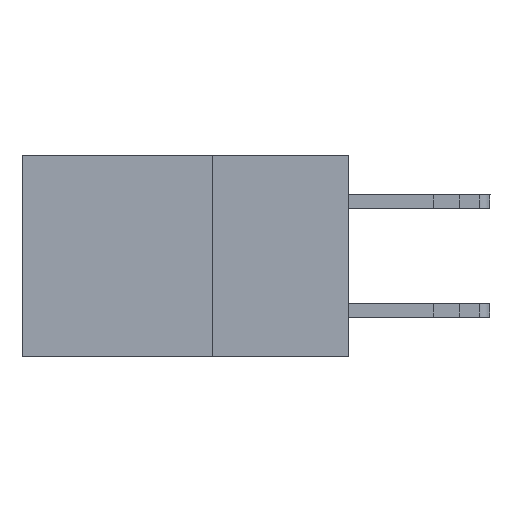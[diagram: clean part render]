
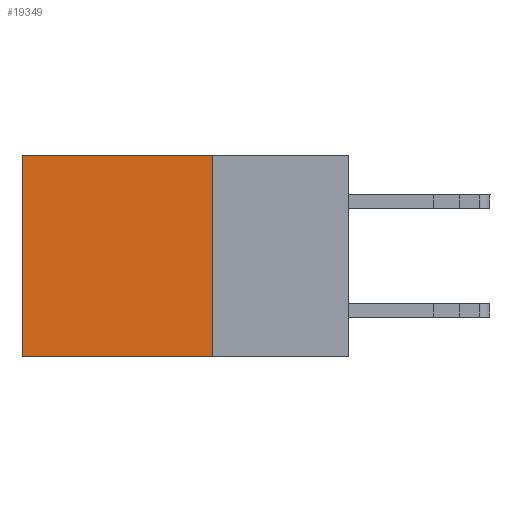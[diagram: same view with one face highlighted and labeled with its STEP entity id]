
A CAD part, left-side view. The second image highlights one B-rep face of the part: STEP entity #19349.
In plain terms, the highlighted planar face has unit normal (-1, 0, 0).
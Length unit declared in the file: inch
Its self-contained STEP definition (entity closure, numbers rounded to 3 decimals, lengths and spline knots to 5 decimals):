
#587 = DIRECTION ( 'NONE',  ( 0., 0., -1. ) ) ;
#704 = EDGE_CURVE ( 'NONE', #1761, #6371, #3309, .T. ) ;
#825 = LINE ( 'NONE', #7078, #16611 ) ;
#1733 = ORIENTED_EDGE ( 'NONE', *, *, #9300, .F. ) ;
#1761 = VERTEX_POINT ( 'NONE', #5199 ) ;
#2770 = LINE ( 'NONE', #9032, #12662 ) ;
#3309 = LINE ( 'NONE', #9355, #19589 ) ;
#5199 = CARTESIAN_POINT ( 'NONE',  ( 0.298, 0.6, 0. ) ) ;
#5217 = PLANE ( 'NONE',  #8790 ) ;
#5387 = CARTESIAN_POINT ( 'NONE',  ( 0.298, 0.25, 0. ) ) ;
#5569 = DIRECTION ( 'NONE',  ( 0., 1., 0. ) ) ;
#5619 = DIRECTION ( 'NONE',  ( 0., 0., -1. ) ) ;
#6371 = VERTEX_POINT ( 'NONE', #6513 ) ;
#6513 = CARTESIAN_POINT ( 'NONE',  ( 0.298, 0.6, -0.37 ) ) ;
#6527 = VERTEX_POINT ( 'NONE', #10358 ) ;
#6856 = DIRECTION ( 'NONE',  ( 0., 0., -1. ) ) ;
#7078 = CARTESIAN_POINT ( 'NONE',  ( 0.298, 0.25, 0. ) ) ;
#7477 = VECTOR ( 'NONE', #5619, 39.37008 ) ;
#7501 = DIRECTION ( 'NONE',  ( 0., 1., 0. ) ) ;
#8781 = EDGE_LOOP ( 'NONE', ( #18501, #1733, #18424, #18123 ) ) ;
#8790 = AXIS2_PLACEMENT_3D ( 'NONE', #11461, #17628, #6856 ) ;
#9032 = CARTESIAN_POINT ( 'NONE',  ( 0.298, 0.25, -0.37 ) ) ;
#9300 = EDGE_CURVE ( 'NONE', #14770, #6371, #2770, .T. ) ;
#9355 = CARTESIAN_POINT ( 'NONE',  ( 0.298, 0.6, 0. ) ) ;
#10358 = CARTESIAN_POINT ( 'NONE',  ( 0.298, 0.25, 0. ) ) ;
#11234 = EDGE_CURVE ( 'NONE', #6527, #14770, #19547, .T. ) ;
#11461 = CARTESIAN_POINT ( 'NONE',  ( 0.298, 0.25, 0. ) ) ;
#12662 = VECTOR ( 'NONE', #7501, 39.37008 ) ;
#14770 = VERTEX_POINT ( 'NONE', #19848 ) ;
#16092 = FACE_OUTER_BOUND ( 'NONE', #8781, .T. ) ;
#16611 = VECTOR ( 'NONE', #5569, 39.37008 ) ;
#17628 = DIRECTION ( 'NONE',  ( 1., 0., 0. ) ) ;
#18123 = ORIENTED_EDGE ( 'NONE', *, *, #19057, .T. ) ;
#18424 = ORIENTED_EDGE ( 'NONE', *, *, #11234, .F. ) ;
#18501 = ORIENTED_EDGE ( 'NONE', *, *, #704, .T. ) ;
#19057 = EDGE_CURVE ( 'NONE', #6527, #1761, #825, .T. ) ;
#19349 = ADVANCED_FACE ( 'NONE', ( #16092 ), #5217, .F. ) ;
#19547 = LINE ( 'NONE', #5387, #7477 ) ;
#19589 = VECTOR ( 'NONE', #587, 39.37008 ) ;
#19848 = CARTESIAN_POINT ( 'NONE',  ( 0.298, 0.25, -0.37 ) ) ;
